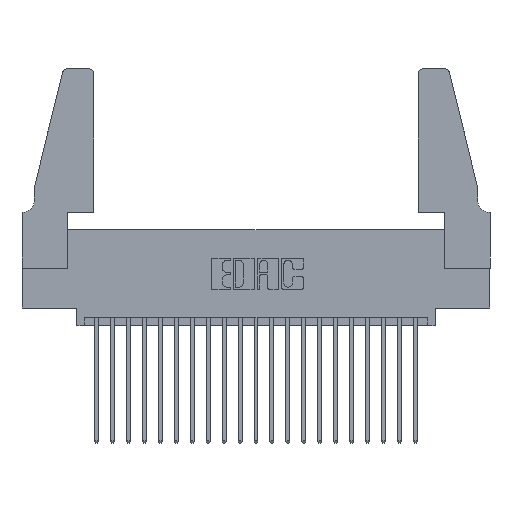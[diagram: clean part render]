
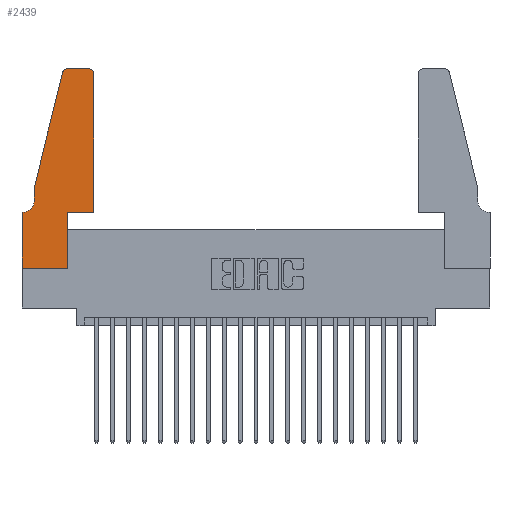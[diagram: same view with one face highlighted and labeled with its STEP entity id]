
A CAD part, top view. The second image highlights one B-rep face of the part: STEP entity #2439.
In plain terms, the highlighted planar face has unit normal (0, 0, 1).
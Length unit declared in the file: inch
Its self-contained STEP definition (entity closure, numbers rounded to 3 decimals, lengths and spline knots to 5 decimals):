
#12 = VECTOR ( 'NONE', #17696, 39.37008 ) ;
#171 = CARTESIAN_POINT ( 'NONE',  ( 0.0055, 0.35, 0.37 ) ) ;
#172 = ORIENTED_EDGE ( 'NONE', *, *, #15469, .T. ) ;
#262 = ORIENTED_EDGE ( 'NONE', *, *, #7107, .T. ) ;
#571 = CARTESIAN_POINT ( 'NONE',  ( 0.4505, 0.35, 0.37 ) ) ;
#608 = CARTESIAN_POINT ( 'NONE',  ( 0., 0., 0.37 ) ) ;
#1055 = ORIENTED_EDGE ( 'NONE', *, *, #2673, .T. ) ;
#1371 = VERTEX_POINT ( 'NONE', #8570 ) ;
#1529 = CARTESIAN_POINT ( 'NONE',  ( 0.2865, 0., 0.37 ) ) ;
#1977 = EDGE_CURVE ( 'NONE', #12794, #1371, #3529, .T. ) ;
#2439 = ADVANCED_FACE ( 'NONE', ( #5734 ), #20821, .T. ) ;
#2517 = DIRECTION ( 'NONE',  ( 1., 0., 0. ) ) ;
#2673 = EDGE_CURVE ( 'NONE', #10583, #12794, #11235, .T. ) ;
#2935 = ORIENTED_EDGE ( 'NONE', *, *, #8209, .T. ) ;
#3368 = VECTOR ( 'NONE', #13075, 39.37008 ) ;
#3529 = LINE ( 'NONE', #16204, #3767 ) ;
#3572 = CARTESIAN_POINT ( 'NONE',  ( 0.4505, 1.22, 0.37 ) ) ;
#3767 = VECTOR ( 'NONE', #18016, 39.37008 ) ;
#4030 = VECTOR ( 'NONE', #12283, 39.37008 ) ;
#4159 = CARTESIAN_POINT ( 'NONE',  ( 0.2605, 1.25, 0.37 ) ) ;
#4216 = EDGE_CURVE ( 'NONE', #9414, #11908, #19784, .T. ) ;
#4561 = DIRECTION ( 'NONE',  ( -1., 0., 0. ) ) ;
#5266 = DIRECTION ( 'NONE',  ( -1., 0., 0. ) ) ;
#5367 = CARTESIAN_POINT ( 'NONE',  ( 0.284, 1.22, 0.37 ) ) ;
#5381 = VERTEX_POINT ( 'NONE', #171 ) ;
#5432 = DIRECTION ( 'NONE',  ( 0., 0., 1. ) ) ;
#5734 = FACE_OUTER_BOUND ( 'NONE', #11361, .T. ) ;
#5784 = VECTOR ( 'NONE', #7273, 39.37008 ) ;
#5874 = AXIS2_PLACEMENT_3D ( 'NONE', #5367, #5432, #20624 ) ;
#6226 = EDGE_CURVE ( 'NONE', #5381, #11580, #17045, .T. ) ;
#6323 = LINE ( 'NONE', #9624, #12 ) ;
#6413 = EDGE_CURVE ( 'NONE', #1371, #9042, #16293, .T. ) ;
#6490 = VERTEX_POINT ( 'NONE', #13019 ) ;
#6673 = EDGE_CURVE ( 'NONE', #11617, #16136, #18349, .T. ) ;
#7029 = CARTESIAN_POINT ( 'NONE',  ( 0., 0.35, 0.37 ) ) ;
#7053 = CARTESIAN_POINT ( 'NONE',  ( 0.4505, 0.35, 0.37 ) ) ;
#7107 = EDGE_CURVE ( 'NONE', #11580, #10583, #11798, .T. ) ;
#7273 = DIRECTION ( 'NONE',  ( 0., -1., 0. ) ) ;
#7636 = DIRECTION ( 'NONE',  ( 0., 0., 1. ) ) ;
#8209 = EDGE_CURVE ( 'NONE', #11908, #6490, #9499, .T. ) ;
#8570 = CARTESIAN_POINT ( 'NONE',  ( 0.2865, 0.35, 0.37 ) ) ;
#8841 = ORIENTED_EDGE ( 'NONE', *, *, #15985, .T. ) ;
#9016 = CARTESIAN_POINT ( 'NONE',  ( 0.0755, 0.5, 0.37 ) ) ;
#9042 = VERTEX_POINT ( 'NONE', #12973 ) ;
#9133 = EDGE_CURVE ( 'NONE', #9042, #9414, #13699, .T. ) ;
#9414 = VERTEX_POINT ( 'NONE', #3572 ) ;
#9499 = LINE ( 'NONE', #4159, #14679 ) ;
#9624 = CARTESIAN_POINT ( 'NONE',  ( 0.0755, 0.5, 0.37 ) ) ;
#10046 = CARTESIAN_POINT ( 'NONE',  ( 0.4205, 1.25, 0.37 ) ) ;
#10583 = VERTEX_POINT ( 'NONE', #608 ) ;
#10837 = DIRECTION ( 'NONE',  ( 0., 0., 1. ) ) ;
#10987 = EDGE_CURVE ( 'NONE', #16136, #11715, #6323, .T. ) ;
#11235 = LINE ( 'NONE', #14819, #3368 ) ;
#11361 = EDGE_LOOP ( 'NONE', ( #2935, #172, #18956, #20283, #8841, #13418, #262, #1055, #12955, #13415, #17456, #15178 ) ) ;
#11580 = VERTEX_POINT ( 'NONE', #7029 ) ;
#11617 = VERTEX_POINT ( 'NONE', #21321 ) ;
#11715 = VERTEX_POINT ( 'NONE', #21607 ) ;
#11798 = LINE ( 'NONE', #16271, #5784 ) ;
#11837 = CIRCLE ( 'NONE', #14304, 0.07 ) ;
#11908 = VERTEX_POINT ( 'NONE', #10046 ) ;
#12283 = DIRECTION ( 'NONE',  ( 0., 1., 0. ) ) ;
#12609 = VECTOR ( 'NONE', #19506, 39.37008 ) ;
#12636 = VECTOR ( 'NONE', #4561, 39.37008 ) ;
#12761 = DIRECTION ( 'NONE',  ( -1., 0., 0. ) ) ;
#12794 = VERTEX_POINT ( 'NONE', #1529 ) ;
#12955 = ORIENTED_EDGE ( 'NONE', *, *, #1977, .T. ) ;
#12973 = CARTESIAN_POINT ( 'NONE',  ( 0.4505, 0.35, 0.37 ) ) ;
#13019 = CARTESIAN_POINT ( 'NONE',  ( 0.284, 1.25, 0.37 ) ) ;
#13075 = DIRECTION ( 'NONE',  ( 1., 0., 0. ) ) ;
#13249 = AXIS2_PLACEMENT_3D ( 'NONE', #16236, #7636, #19590 ) ;
#13415 = ORIENTED_EDGE ( 'NONE', *, *, #6413, .T. ) ;
#13418 = ORIENTED_EDGE ( 'NONE', *, *, #6226, .T. ) ;
#13594 = DIRECTION ( 'NONE',  ( 0., 0., -1. ) ) ;
#13699 = LINE ( 'NONE', #571, #4030 ) ;
#14304 = AXIS2_PLACEMENT_3D ( 'NONE', #20254, #13594, #5266 ) ;
#14623 = AXIS2_PLACEMENT_3D ( 'NONE', #15590, #10837, #2517 ) ;
#14679 = VECTOR ( 'NONE', #12761, 39.37008 ) ;
#14819 = CARTESIAN_POINT ( 'NONE',  ( 0., 0., 0.37 ) ) ;
#15178 = ORIENTED_EDGE ( 'NONE', *, *, #4216, .T. ) ;
#15469 = EDGE_CURVE ( 'NONE', #6490, #11617, #19466, .T. ) ;
#15590 = CARTESIAN_POINT ( 'NONE',  ( 0., 0.35, 0.37 ) ) ;
#15985 = EDGE_CURVE ( 'NONE', #11715, #5381, #11837, .T. ) ;
#16136 = VERTEX_POINT ( 'NONE', #20457 ) ;
#16204 = CARTESIAN_POINT ( 'NONE',  ( 0.2865, 0.35, 0.37 ) ) ;
#16236 = CARTESIAN_POINT ( 'NONE',  ( 0.4205, 1.22, 0.37 ) ) ;
#16271 = CARTESIAN_POINT ( 'NONE',  ( 0., 0., 0.37 ) ) ;
#16293 = LINE ( 'NONE', #7053, #20699 ) ;
#17045 = LINE ( 'NONE', #17945, #12636 ) ;
#17456 = ORIENTED_EDGE ( 'NONE', *, *, #9133, .T. ) ;
#17696 = DIRECTION ( 'NONE',  ( 0., -1., 0. ) ) ;
#17945 = CARTESIAN_POINT ( 'NONE',  ( 0.0755, 0.35, 0.37 ) ) ;
#18016 = DIRECTION ( 'NONE',  ( 0., 1., 0. ) ) ;
#18349 = LINE ( 'NONE', #9016, #12609 ) ;
#18562 = DIRECTION ( 'NONE',  ( 1., 0., 0. ) ) ;
#18956 = ORIENTED_EDGE ( 'NONE', *, *, #6673, .T. ) ;
#19466 = CIRCLE ( 'NONE', #5874, 0.03 ) ;
#19506 = DIRECTION ( 'NONE',  ( -0.239, -0.971, 0. ) ) ;
#19590 = DIRECTION ( 'NONE',  ( 1., 0., 0. ) ) ;
#19784 = CIRCLE ( 'NONE', #13249, 0.03 ) ;
#20254 = CARTESIAN_POINT ( 'NONE',  ( 0.0055, 0.42, 0.37 ) ) ;
#20283 = ORIENTED_EDGE ( 'NONE', *, *, #10987, .T. ) ;
#20457 = CARTESIAN_POINT ( 'NONE',  ( 0.0755, 0.5, 0.37 ) ) ;
#20624 = DIRECTION ( 'NONE',  ( 1., 0., 0. ) ) ;
#20699 = VECTOR ( 'NONE', #18562, 39.37008 ) ;
#20821 = PLANE ( 'NONE',  #14623 ) ;
#21321 = CARTESIAN_POINT ( 'NONE',  ( 0.25487, 1.22718, 0.37 ) ) ;
#21607 = CARTESIAN_POINT ( 'NONE',  ( 0.0755, 0.42, 0.37 ) ) ;
